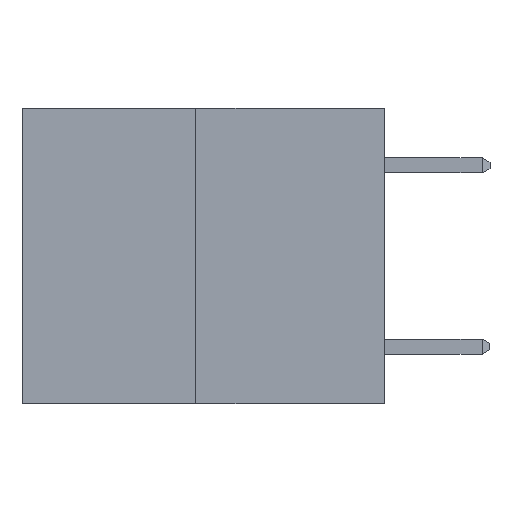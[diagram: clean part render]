
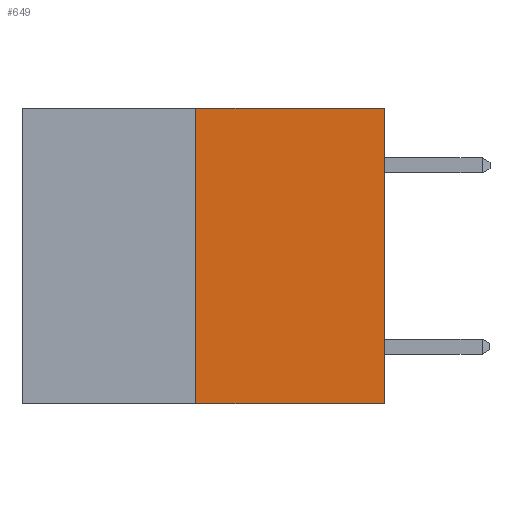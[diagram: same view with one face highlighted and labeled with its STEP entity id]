
A CAD part, left-side view. The second image highlights one B-rep face of the part: STEP entity #649.
In plain terms, the highlighted planar face has unit normal (-1, 0, 0).
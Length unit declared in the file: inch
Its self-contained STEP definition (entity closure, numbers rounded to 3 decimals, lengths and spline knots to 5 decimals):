
#163 = VECTOR ( 'NONE', #4188, 39.37008 ) ;
#190 = DIRECTION ( 'NONE',  ( 0., -1., 0. ) ) ;
#299 = EDGE_CURVE ( 'NONE', #15057, #11098, #6693, .T. ) ;
#372 = CARTESIAN_POINT ( 'NONE',  ( 0., 0., 0. ) ) ;
#649 = ADVANCED_FACE ( 'NONE', ( #3881 ), #1107, .F. ) ;
#742 = EDGE_LOOP ( 'NONE', ( #4647, #8202, #4496, #1555 ) ) ;
#1107 = PLANE ( 'NONE',  #14528 ) ;
#1555 = ORIENTED_EDGE ( 'NONE', *, *, #12622, .F. ) ;
#1623 = DIRECTION ( 'NONE',  ( 0., 0., 1. ) ) ;
#3588 = EDGE_CURVE ( 'NONE', #11098, #6195, #8752, .T. ) ;
#3881 = FACE_OUTER_BOUND ( 'NONE', #742, .T. ) ;
#4101 = CARTESIAN_POINT ( 'NONE',  ( 0., 0., -0.49 ) ) ;
#4188 = DIRECTION ( 'NONE',  ( 0., -1., 0. ) ) ;
#4256 = CARTESIAN_POINT ( 'NONE',  ( 0., 0.312, -0.49 ) ) ;
#4496 = ORIENTED_EDGE ( 'NONE', *, *, #3588, .T. ) ;
#4647 = ORIENTED_EDGE ( 'NONE', *, *, #14132, .F. ) ;
#6192 = VERTEX_POINT ( 'NONE', #6993 ) ;
#6195 = VERTEX_POINT ( 'NONE', #11781 ) ;
#6693 = LINE ( 'NONE', #14426, #14543 ) ;
#6993 = CARTESIAN_POINT ( 'NONE',  ( 0., 0.312, 0. ) ) ;
#7301 = VECTOR ( 'NONE', #9364, 39.37008 ) ;
#7679 = LINE ( 'NONE', #10592, #7301 ) ;
#8202 = ORIENTED_EDGE ( 'NONE', *, *, #299, .T. ) ;
#8752 = LINE ( 'NONE', #372, #11000 ) ;
#9251 = DIRECTION ( 'NONE',  ( 0., 0., -1. ) ) ;
#9364 = DIRECTION ( 'NONE',  ( 0., 0., 1. ) ) ;
#10495 = DIRECTION ( 'NONE',  ( 1., 0., 0. ) ) ;
#10592 = CARTESIAN_POINT ( 'NONE',  ( 0., 0.312, -0.49 ) ) ;
#11000 = VECTOR ( 'NONE', #1623, 39.37008 ) ;
#11098 = VERTEX_POINT ( 'NONE', #4101 ) ;
#11286 = LINE ( 'NONE', #12554, #163 ) ;
#11537 = CARTESIAN_POINT ( 'NONE',  ( 0., 0.6, 0. ) ) ;
#11781 = CARTESIAN_POINT ( 'NONE',  ( 0., 0., 0. ) ) ;
#12554 = CARTESIAN_POINT ( 'NONE',  ( 0., 0.6, 0. ) ) ;
#12622 = EDGE_CURVE ( 'NONE', #6192, #6195, #11286, .T. ) ;
#14132 = EDGE_CURVE ( 'NONE', #15057, #6192, #7679, .T. ) ;
#14426 = CARTESIAN_POINT ( 'NONE',  ( 0., 0.6, -0.49 ) ) ;
#14528 = AXIS2_PLACEMENT_3D ( 'NONE', #11537, #10495, #9251 ) ;
#14543 = VECTOR ( 'NONE', #190, 39.37008 ) ;
#15057 = VERTEX_POINT ( 'NONE', #4256 ) ;
